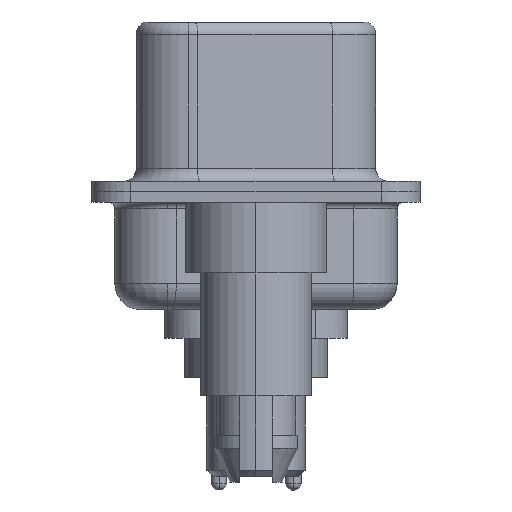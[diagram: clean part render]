
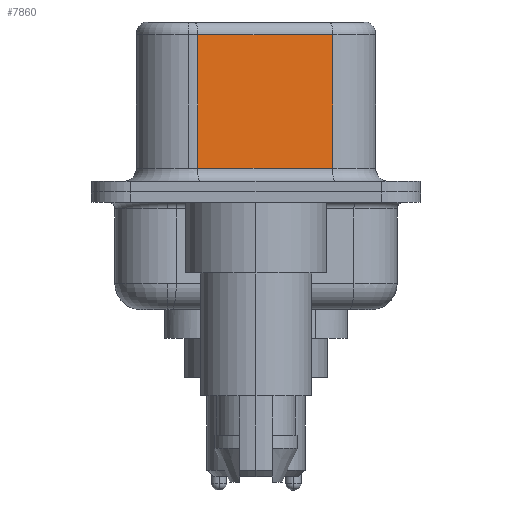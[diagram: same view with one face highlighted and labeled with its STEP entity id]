
A CAD part, left-side view. The second image highlights one B-rep face of the part: STEP entity #7860.
In plain terms, the highlighted planar face has unit normal (-0.985, -0.174, 0).
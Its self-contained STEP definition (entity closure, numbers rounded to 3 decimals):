
#1148 = EDGE_CURVE ( 'NONE', #14066, #10576, #20943, .T. ) ;
#1508 = DIRECTION ( 'NONE',  ( 0., 0., -1. ) ) ;
#1678 = CARTESIAN_POINT ( 'NONE',  ( 4.585, -2.927, 0.9 ) ) ;
#1828 = VECTOR ( 'NONE', #1508, 1000. ) ;
#3890 = EDGE_CURVE ( 'NONE', #16282, #10576, #14960, .T. ) ;
#4020 = LINE ( 'NONE', #22188, #22025 ) ;
#4509 = PLANE ( 'NONE',  #17857 ) ;
#6303 = DIRECTION ( 'NONE',  ( 0.985, 0.174, 0. ) ) ;
#6358 = CARTESIAN_POINT ( 'NONE',  ( 4.585, -2.927, 6.52 ) ) ;
#7651 = CARTESIAN_POINT ( 'NONE',  ( 4.585, -2.927, 6.02 ) ) ;
#7860 = ADVANCED_FACE ( 'NONE', ( #13250 ), #4509, .F. ) ;
#7904 = LINE ( 'NONE', #22578, #11509 ) ;
#10170 = VECTOR ( 'NONE', #15861, 1000. ) ;
#10576 = VERTEX_POINT ( 'NONE', #18128 ) ;
#10900 = VERTEX_POINT ( 'NONE', #11650 ) ;
#11339 = DIRECTION ( 'NONE',  ( -0.174, 0.985, 0. ) ) ;
#11509 = VECTOR ( 'NONE', #13566, 1000. ) ;
#11650 = CARTESIAN_POINT ( 'NONE',  ( 3.675, 2.233, 6.02 ) ) ;
#13250 = FACE_OUTER_BOUND ( 'NONE', #21975, .T. ) ;
#13412 = CARTESIAN_POINT ( 'NONE',  ( 4.585, -2.927, 6.52 ) ) ;
#13566 = DIRECTION ( 'NONE',  ( 0., 0., -1. ) ) ;
#14066 = VERTEX_POINT ( 'NONE', #7651 ) ;
#14538 = ORIENTED_EDGE ( 'NONE', *, *, #1148, .F. ) ;
#14845 = EDGE_CURVE ( 'NONE', #10900, #16282, #7904, .T. ) ;
#14960 = LINE ( 'NONE', #1678, #10170 ) ;
#15861 = DIRECTION ( 'NONE',  ( 0.174, -0.985, 0. ) ) ;
#16282 = VERTEX_POINT ( 'NONE', #23040 ) ;
#17857 = AXIS2_PLACEMENT_3D ( 'NONE', #13412, #6303, #18809 ) ;
#18128 = CARTESIAN_POINT ( 'NONE',  ( 4.585, -2.927, 0.9 ) ) ;
#18809 = DIRECTION ( 'NONE',  ( -0.174, 0.985, 0. ) ) ;
#20474 = ORIENTED_EDGE ( 'NONE', *, *, #14845, .T. ) ;
#20943 = LINE ( 'NONE', #6358, #1828 ) ;
#21145 = ORIENTED_EDGE ( 'NONE', *, *, #3890, .T. ) ;
#21552 = EDGE_CURVE ( 'NONE', #14066, #10900, #4020, .T. ) ;
#21975 = EDGE_LOOP ( 'NONE', ( #14538, #22866, #20474, #21145 ) ) ;
#22025 = VECTOR ( 'NONE', #11339, 1000. ) ;
#22188 = CARTESIAN_POINT ( 'NONE',  ( 4.585, -2.927, 6.02 ) ) ;
#22578 = CARTESIAN_POINT ( 'NONE',  ( 3.675, 2.233, 6.52 ) ) ;
#22866 = ORIENTED_EDGE ( 'NONE', *, *, #21552, .T. ) ;
#23040 = CARTESIAN_POINT ( 'NONE',  ( 3.675, 2.233, 0.9 ) ) ;
